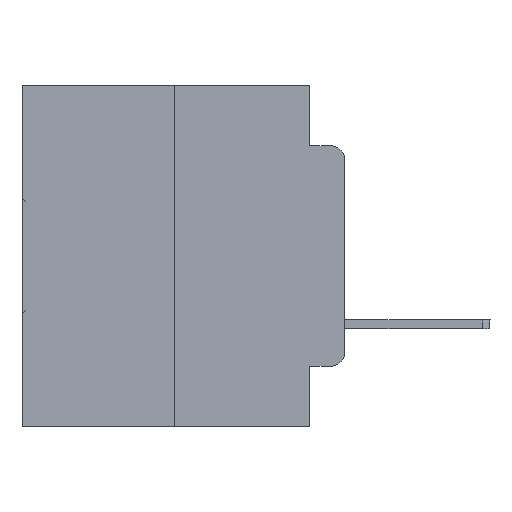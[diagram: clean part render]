
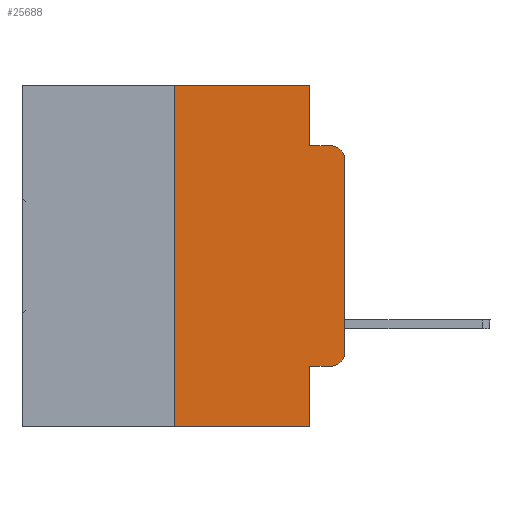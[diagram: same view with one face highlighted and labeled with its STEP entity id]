
A CAD part, left-side view. The second image highlights one B-rep face of the part: STEP entity #25688.
In plain terms, the highlighted planar face has unit normal (-1, 0, 0).
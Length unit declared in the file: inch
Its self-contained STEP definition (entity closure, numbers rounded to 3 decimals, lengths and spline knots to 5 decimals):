
#243 = DIRECTION ( 'NONE',  ( 0., 0., -1. ) ) ;
#575 = CARTESIAN_POINT ( 'NONE',  ( 0., 0.02, -0.4115 ) ) ;
#881 = ORIENTED_EDGE ( 'NONE', *, *, #12864, .F. ) ;
#974 = VERTEX_POINT ( 'NONE', #18692 ) ;
#1075 = EDGE_CURVE ( 'NONE', #974, #25345, #30565, .T. ) ;
#1806 = EDGE_CURVE ( 'NONE', #13595, #13604, #6821, .T. ) ;
#2096 = CARTESIAN_POINT ( 'NONE',  ( 0., 0., 0. ) ) ;
#2322 = AXIS2_PLACEMENT_3D ( 'NONE', #5474, #15145, #26214 ) ;
#2554 = DIRECTION ( 'NONE',  ( 0., 0., 1. ) ) ;
#3361 = CIRCLE ( 'NONE', #4385, 0.02 ) ;
#3713 = DIRECTION ( 'NONE',  ( 0., 0., 1. ) ) ;
#3904 = DIRECTION ( 'NONE',  ( 0., -1., 0. ) ) ;
#3943 = LINE ( 'NONE', #23571, #6133 ) ;
#4116 = EDGE_LOOP ( 'NONE', ( #16831, #5409, #26671, #13438, #21795, #881, #15684, #25263, #12918, #12682 ) ) ;
#4385 = AXIS2_PLACEMENT_3D ( 'NONE', #7360, #7206, #243 ) ;
#5409 = ORIENTED_EDGE ( 'NONE', *, *, #1806, .T. ) ;
#5474 = CARTESIAN_POINT ( 'NONE',  ( 0., 0.02, -0.1085 ) ) ;
#6133 = VECTOR ( 'NONE', #27840, 39.37008 ) ;
#6215 = LINE ( 'NONE', #15556, #19640 ) ;
#6642 = VERTEX_POINT ( 'NONE', #575 ) ;
#6821 = CIRCLE ( 'NONE', #2322, 0.02 ) ;
#7206 = DIRECTION ( 'NONE',  ( -1., 0., 0. ) ) ;
#7360 = CARTESIAN_POINT ( 'NONE',  ( 0., 0.02, -0.3915 ) ) ;
#8495 = LINE ( 'NONE', #10705, #16577 ) ;
#8972 = CARTESIAN_POINT ( 'NONE',  ( 0., 0.473, 0. ) ) ;
#9730 = CARTESIAN_POINT ( 'NONE',  ( 0., 0.051, 0. ) ) ;
#10705 = CARTESIAN_POINT ( 'NONE',  ( 0., 0.051, -0.4115 ) ) ;
#11109 = EDGE_CURVE ( 'NONE', #15226, #15479, #28264, .T. ) ;
#11196 = CARTESIAN_POINT ( 'NONE',  ( 0., 0., -0.3915 ) ) ;
#11392 = VECTOR ( 'NONE', #3713, 39.37008 ) ;
#11984 = EDGE_CURVE ( 'NONE', #25308, #25345, #3943, .T. ) ;
#11995 = EDGE_CURVE ( 'NONE', #13192, #13604, #18495, .T. ) ;
#12682 = ORIENTED_EDGE ( 'NONE', *, *, #15423, .T. ) ;
#12864 = EDGE_CURVE ( 'NONE', #974, #15226, #13840, .T. ) ;
#12918 = ORIENTED_EDGE ( 'NONE', *, *, #17021, .T. ) ;
#13192 = VERTEX_POINT ( 'NONE', #24417 ) ;
#13438 = ORIENTED_EDGE ( 'NONE', *, *, #29529, .F. ) ;
#13595 = VERTEX_POINT ( 'NONE', #29584 ) ;
#13604 = VERTEX_POINT ( 'NONE', #17245 ) ;
#13763 = CARTESIAN_POINT ( 'NONE',  ( 0., 0.051, -0.0885 ) ) ;
#13840 = LINE ( 'NONE', #25403, #11392 ) ;
#14065 = CARTESIAN_POINT ( 'NONE',  ( 0., 0.051, -0.4115 ) ) ;
#15145 = DIRECTION ( 'NONE',  ( -1., 0., 0. ) ) ;
#15226 = VERTEX_POINT ( 'NONE', #29560 ) ;
#15423 = EDGE_CURVE ( 'NONE', #6642, #20892, #3361, .T. ) ;
#15479 = VERTEX_POINT ( 'NONE', #9730 ) ;
#15556 = CARTESIAN_POINT ( 'NONE',  ( 0., 0.051, 0. ) ) ;
#15684 = ORIENTED_EDGE ( 'NONE', *, *, #1075, .T. ) ;
#16577 = VECTOR ( 'NONE', #20347, 39.37008 ) ;
#16831 = ORIENTED_EDGE ( 'NONE', *, *, #26122, .T. ) ;
#17021 = EDGE_CURVE ( 'NONE', #25308, #6642, #8495, .T. ) ;
#17245 = CARTESIAN_POINT ( 'NONE',  ( 0., 0.02, -0.0885 ) ) ;
#17792 = CARTESIAN_POINT ( 'NONE',  ( 0., 0.051, -0.5 ) ) ;
#18495 = LINE ( 'NONE', #13763, #26892 ) ;
#18692 = CARTESIAN_POINT ( 'NONE',  ( 0., 0.25, -0.5 ) ) ;
#19351 = FACE_OUTER_BOUND ( 'NONE', #4116, .T. ) ;
#19640 = VECTOR ( 'NONE', #25682, 39.37008 ) ;
#20347 = DIRECTION ( 'NONE',  ( 0., -1., 0. ) ) ;
#20892 = VERTEX_POINT ( 'NONE', #11196 ) ;
#21178 = VECTOR ( 'NONE', #3904, 39.37008 ) ;
#21275 = PLANE ( 'NONE',  #25132 ) ;
#21466 = VECTOR ( 'NONE', #23612, 39.37008 ) ;
#21795 = ORIENTED_EDGE ( 'NONE', *, *, #11109, .F. ) ;
#23415 = DIRECTION ( 'NONE',  ( 0., -1., 0. ) ) ;
#23571 = CARTESIAN_POINT ( 'NONE',  ( 0., 0.051, 0. ) ) ;
#23612 = DIRECTION ( 'NONE',  ( 0., -1., 0. ) ) ;
#24221 = LINE ( 'NONE', #2096, #26160 ) ;
#24417 = CARTESIAN_POINT ( 'NONE',  ( 0., 0.051, -0.0885 ) ) ;
#25132 = AXIS2_PLACEMENT_3D ( 'NONE', #31075, #29011, #28699 ) ;
#25263 = ORIENTED_EDGE ( 'NONE', *, *, #11984, .F. ) ;
#25308 = VERTEX_POINT ( 'NONE', #14065 ) ;
#25345 = VERTEX_POINT ( 'NONE', #17792 ) ;
#25403 = CARTESIAN_POINT ( 'NONE',  ( 0., 0.25, 0. ) ) ;
#25682 = DIRECTION ( 'NONE',  ( 0., 0., -1. ) ) ;
#25688 = ADVANCED_FACE ( 'NONE', ( #19351 ), #21275, .F. ) ;
#26122 = EDGE_CURVE ( 'NONE', #20892, #13595, #24221, .T. ) ;
#26160 = VECTOR ( 'NONE', #2554, 39.37008 ) ;
#26214 = DIRECTION ( 'NONE',  ( 0., 0., -1. ) ) ;
#26671 = ORIENTED_EDGE ( 'NONE', *, *, #11995, .F. ) ;
#26892 = VECTOR ( 'NONE', #23415, 39.37008 ) ;
#27840 = DIRECTION ( 'NONE',  ( 0., 0., -1. ) ) ;
#28264 = LINE ( 'NONE', #8972, #21178 ) ;
#28699 = DIRECTION ( 'NONE',  ( 0., 0., -1. ) ) ;
#28818 = CARTESIAN_POINT ( 'NONE',  ( 0., 0.473, -0.5 ) ) ;
#29011 = DIRECTION ( 'NONE',  ( 1., 0., 0. ) ) ;
#29529 = EDGE_CURVE ( 'NONE', #15479, #13192, #6215, .T. ) ;
#29560 = CARTESIAN_POINT ( 'NONE',  ( 0., 0.25, 0. ) ) ;
#29584 = CARTESIAN_POINT ( 'NONE',  ( 0., 0., -0.1085 ) ) ;
#30565 = LINE ( 'NONE', #28818, #21466 ) ;
#31075 = CARTESIAN_POINT ( 'NONE',  ( 0., 0.473, 0. ) ) ;
